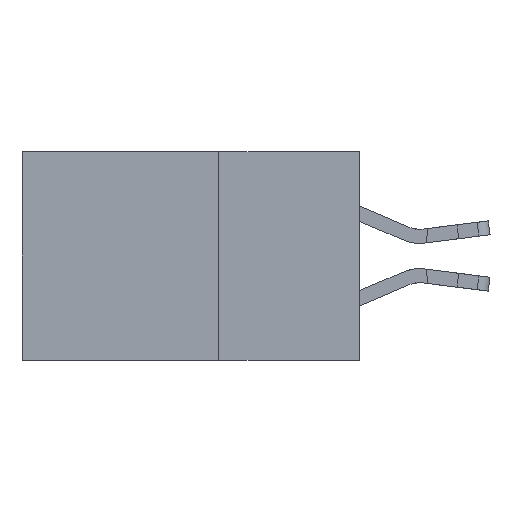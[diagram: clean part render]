
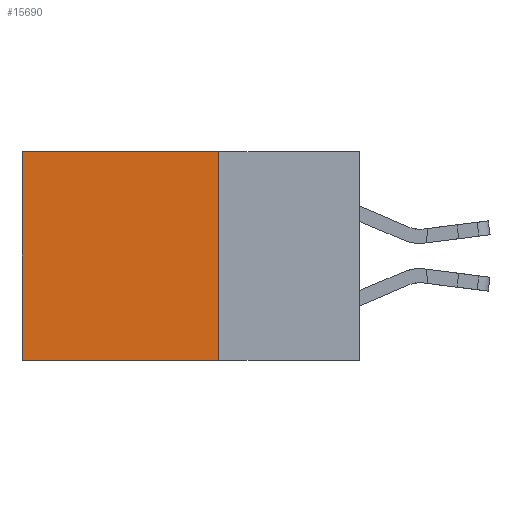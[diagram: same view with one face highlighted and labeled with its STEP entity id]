
A CAD part, left-side view. The second image highlights one B-rep face of the part: STEP entity #15690.
In plain terms, the highlighted planar face has unit normal (-1, 0, 0).
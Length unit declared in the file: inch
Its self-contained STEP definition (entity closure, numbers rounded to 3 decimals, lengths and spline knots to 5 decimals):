
#37 = ORIENTED_EDGE ( 'NONE', *, *, #7268, .F. ) ;
#506 = VECTOR ( 'NONE', #4574, 39.37008 ) ;
#554 = ORIENTED_EDGE ( 'NONE', *, *, #4684, .F. ) ;
#588 = CARTESIAN_POINT ( 'NONE',  ( 0.2875, 0.6, 0. ) ) ;
#852 = EDGE_LOOP ( 'NONE', ( #19466, #37, #554, #12796 ) ) ;
#1889 = LINE ( 'NONE', #23264, #7025 ) ;
#2243 = CARTESIAN_POINT ( 'NONE',  ( 0.2875, 0.6, 0. ) ) ;
#3530 = EDGE_CURVE ( 'NONE', #8175, #22574, #1889, .T. ) ;
#3901 = DIRECTION ( 'NONE',  ( 0., 0., -1. ) ) ;
#4226 = LINE ( 'NONE', #20741, #506 ) ;
#4574 = DIRECTION ( 'NONE',  ( 0., 0., -1. ) ) ;
#4684 = EDGE_CURVE ( 'NONE', #8175, #8187, #4226, .T. ) ;
#5396 = EDGE_CURVE ( 'NONE', #22574, #23163, #20081, .T. ) ;
#5670 = VECTOR ( 'NONE', #3901, 39.37008 ) ;
#7025 = VECTOR ( 'NONE', #10649, 39.37008 ) ;
#7268 = EDGE_CURVE ( 'NONE', #8187, #23163, #11649, .T. ) ;
#8175 = VERTEX_POINT ( 'NONE', #13394 ) ;
#8187 = VERTEX_POINT ( 'NONE', #22601 ) ;
#10649 = DIRECTION ( 'NONE',  ( 0., 1., 0. ) ) ;
#11649 = LINE ( 'NONE', #20976, #21915 ) ;
#11783 = CARTESIAN_POINT ( 'NONE',  ( 0.2875, 0.6, -0.37 ) ) ;
#11794 = PLANE ( 'NONE',  #12747 ) ;
#12747 = AXIS2_PLACEMENT_3D ( 'NONE', #18985, #20649, #15314 ) ;
#12796 = ORIENTED_EDGE ( 'NONE', *, *, #3530, .T. ) ;
#13394 = CARTESIAN_POINT ( 'NONE',  ( 0.2875, 0.25, 0. ) ) ;
#14774 = FACE_OUTER_BOUND ( 'NONE', #852, .T. ) ;
#15314 = DIRECTION ( 'NONE',  ( 0., 0., -1. ) ) ;
#15690 = ADVANCED_FACE ( 'NONE', ( #14774 ), #11794, .F. ) ;
#18853 = DIRECTION ( 'NONE',  ( 0., 1., 0. ) ) ;
#18985 = CARTESIAN_POINT ( 'NONE',  ( 0.2875, 0.25, 0. ) ) ;
#19466 = ORIENTED_EDGE ( 'NONE', *, *, #5396, .T. ) ;
#20081 = LINE ( 'NONE', #588, #5670 ) ;
#20649 = DIRECTION ( 'NONE',  ( 1., 0., 0. ) ) ;
#20741 = CARTESIAN_POINT ( 'NONE',  ( 0.2875, 0.25, 0. ) ) ;
#20976 = CARTESIAN_POINT ( 'NONE',  ( 0.2875, 0.25, -0.37 ) ) ;
#21915 = VECTOR ( 'NONE', #18853, 39.37008 ) ;
#22574 = VERTEX_POINT ( 'NONE', #2243 ) ;
#22601 = CARTESIAN_POINT ( 'NONE',  ( 0.2875, 0.25, -0.37 ) ) ;
#23163 = VERTEX_POINT ( 'NONE', #11783 ) ;
#23264 = CARTESIAN_POINT ( 'NONE',  ( 0.2875, 0.25, 0. ) ) ;
